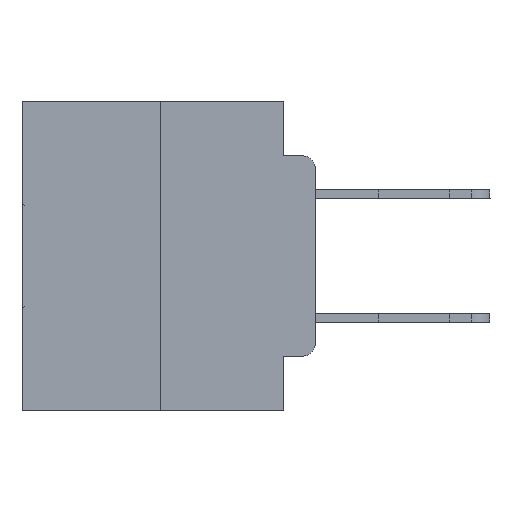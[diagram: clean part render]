
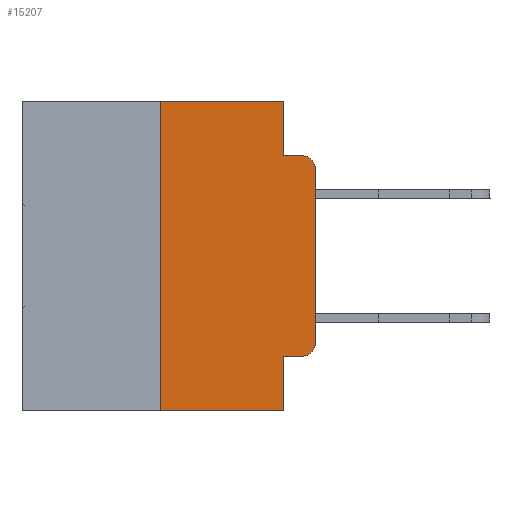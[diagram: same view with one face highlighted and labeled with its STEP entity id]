
A CAD part, left-side view. The second image highlights one B-rep face of the part: STEP entity #15207.
In plain terms, the highlighted planar face has unit normal (-1, 0, 0).
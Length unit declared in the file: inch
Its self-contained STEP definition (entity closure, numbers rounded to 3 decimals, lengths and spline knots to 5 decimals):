
#726 = DIRECTION ( 'NONE',  ( 0., 0., -1. ) ) ;
#745 = ORIENTED_EDGE ( 'NONE', *, *, #25341, .F. ) ;
#1807 = CARTESIAN_POINT ( 'NONE',  ( 0., 0.25, 0. ) ) ;
#2274 = ORIENTED_EDGE ( 'NONE', *, *, #5739, .F. ) ;
#2946 = VECTOR ( 'NONE', #726, 39.37008 ) ;
#3350 = CARTESIAN_POINT ( 'NONE',  ( 0., 0., 0. ) ) ;
#3655 = VECTOR ( 'NONE', #16462, 39.37008 ) ;
#3758 = VERTEX_POINT ( 'NONE', #6797 ) ;
#4057 = EDGE_CURVE ( 'NONE', #8524, #8776, #22356, .T. ) ;
#4253 = LINE ( 'NONE', #29282, #29813 ) ;
#4266 = VERTEX_POINT ( 'NONE', #20864 ) ;
#4558 = EDGE_LOOP ( 'NONE', ( #22821, #4998, #11525, #25002, #745, #2274, #21728, #22476, #28677, #23927 ) ) ;
#4998 = ORIENTED_EDGE ( 'NONE', *, *, #12325, .T. ) ;
#5038 = VECTOR ( 'NONE', #22798, 39.37008 ) ;
#5739 = EDGE_CURVE ( 'NONE', #27080, #23513, #28516, .T. ) ;
#6314 = VERTEX_POINT ( 'NONE', #9433 ) ;
#6797 = CARTESIAN_POINT ( 'NONE',  ( 0., 0., -0.1085 ) ) ;
#6836 = AXIS2_PLACEMENT_3D ( 'NONE', #23693, #9259, #26012 ) ;
#7069 = LINE ( 'NONE', #26354, #19217 ) ;
#7763 = DIRECTION ( 'NONE',  ( 0., 0., -1. ) ) ;
#7784 = CIRCLE ( 'NONE', #6836, 0.02 ) ;
#8524 = VERTEX_POINT ( 'NONE', #25111 ) ;
#8709 = CARTESIAN_POINT ( 'NONE',  ( 0., 0.051, -0.0885 ) ) ;
#8776 = VERTEX_POINT ( 'NONE', #26008 ) ;
#9035 = EDGE_CURVE ( 'NONE', #16711, #6314, #4253, .T. ) ;
#9223 = AXIS2_PLACEMENT_3D ( 'NONE', #10762, #13210, #29814 ) ;
#9259 = DIRECTION ( 'NONE',  ( -1., 0., 0. ) ) ;
#9404 = DIRECTION ( 'NONE',  ( 0., -1., 0. ) ) ;
#9433 = CARTESIAN_POINT ( 'NONE',  ( 0., 0.051, -0.0885 ) ) ;
#10379 = VERTEX_POINT ( 'NONE', #17239 ) ;
#10684 = EDGE_CURVE ( 'NONE', #6314, #4266, #16758, .T. ) ;
#10762 = CARTESIAN_POINT ( 'NONE',  ( 0., 0.473, 0. ) ) ;
#11124 = CARTESIAN_POINT ( 'NONE',  ( 0., 0.051, 0. ) ) ;
#11525 = ORIENTED_EDGE ( 'NONE', *, *, #10684, .F. ) ;
#12325 = EDGE_CURVE ( 'NONE', #3758, #4266, #22347, .T. ) ;
#12922 = DIRECTION ( 'NONE',  ( -1., 0., 0. ) ) ;
#13210 = DIRECTION ( 'NONE',  ( 1., 0., 0. ) ) ;
#14292 = CARTESIAN_POINT ( 'NONE',  ( 0., 0.473, -0.5 ) ) ;
#15207 = ADVANCED_FACE ( 'NONE', ( #30270 ), #15519, .F. ) ;
#15519 = PLANE ( 'NONE',  #9223 ) ;
#15844 = CARTESIAN_POINT ( 'NONE',  ( 0., 0.25, 0. ) ) ;
#16055 = CARTESIAN_POINT ( 'NONE',  ( 0., 0.051, -0.4115 ) ) ;
#16462 = DIRECTION ( 'NONE',  ( 0., 0., 1. ) ) ;
#16711 = VERTEX_POINT ( 'NONE', #11124 ) ;
#16758 = LINE ( 'NONE', #8709, #27145 ) ;
#17174 = EDGE_CURVE ( 'NONE', #10379, #3758, #30533, .T. ) ;
#17239 = CARTESIAN_POINT ( 'NONE',  ( 0., 0., -0.3915 ) ) ;
#17476 = VECTOR ( 'NONE', #9404, 39.37008 ) ;
#19211 = EDGE_CURVE ( 'NONE', #27080, #8776, #30023, .T. ) ;
#19217 = VECTOR ( 'NONE', #28713, 39.37008 ) ;
#20811 = AXIS2_PLACEMENT_3D ( 'NONE', #26765, #12922, #29520 ) ;
#20864 = CARTESIAN_POINT ( 'NONE',  ( 0., 0.02, -0.0885 ) ) ;
#21728 = ORIENTED_EDGE ( 'NONE', *, *, #19211, .T. ) ;
#22347 = CIRCLE ( 'NONE', #20811, 0.02 ) ;
#22356 = LINE ( 'NONE', #24877, #2946 ) ;
#22476 = ORIENTED_EDGE ( 'NONE', *, *, #4057, .F. ) ;
#22798 = DIRECTION ( 'NONE',  ( 0., 0., 1. ) ) ;
#22821 = ORIENTED_EDGE ( 'NONE', *, *, #17174, .T. ) ;
#23177 = DIRECTION ( 'NONE',  ( 0., -1., 0. ) ) ;
#23280 = DIRECTION ( 'NONE',  ( 0., -1., 0. ) ) ;
#23513 = VERTEX_POINT ( 'NONE', #15844 ) ;
#23693 = CARTESIAN_POINT ( 'NONE',  ( 0., 0.02, -0.3915 ) ) ;
#23789 = CARTESIAN_POINT ( 'NONE',  ( 0., 0.02, -0.4115 ) ) ;
#23927 = ORIENTED_EDGE ( 'NONE', *, *, #28851, .T. ) ;
#24247 = VECTOR ( 'NONE', #23280, 39.37008 ) ;
#24877 = CARTESIAN_POINT ( 'NONE',  ( 0., 0.051, 0. ) ) ;
#25002 = ORIENTED_EDGE ( 'NONE', *, *, #9035, .F. ) ;
#25111 = CARTESIAN_POINT ( 'NONE',  ( 0., 0.051, -0.4115 ) ) ;
#25341 = EDGE_CURVE ( 'NONE', #23513, #16711, #7069, .T. ) ;
#25878 = CARTESIAN_POINT ( 'NONE',  ( 0., 0.25, -0.5 ) ) ;
#26008 = CARTESIAN_POINT ( 'NONE',  ( 0., 0.051, -0.5 ) ) ;
#26012 = DIRECTION ( 'NONE',  ( 0., 0., -1. ) ) ;
#26354 = CARTESIAN_POINT ( 'NONE',  ( 0., 0.473, 0. ) ) ;
#26765 = CARTESIAN_POINT ( 'NONE',  ( 0., 0.02, -0.1085 ) ) ;
#27080 = VERTEX_POINT ( 'NONE', #25878 ) ;
#27145 = VECTOR ( 'NONE', #23177, 39.37008 ) ;
#28516 = LINE ( 'NONE', #1807, #3655 ) ;
#28677 = ORIENTED_EDGE ( 'NONE', *, *, #30417, .T. ) ;
#28713 = DIRECTION ( 'NONE',  ( 0., -1., 0. ) ) ;
#28851 = EDGE_CURVE ( 'NONE', #28881, #10379, #7784, .T. ) ;
#28881 = VERTEX_POINT ( 'NONE', #23789 ) ;
#29282 = CARTESIAN_POINT ( 'NONE',  ( 0., 0.051, 0. ) ) ;
#29520 = DIRECTION ( 'NONE',  ( 0., 0., -1. ) ) ;
#29813 = VECTOR ( 'NONE', #7763, 39.37008 ) ;
#29814 = DIRECTION ( 'NONE',  ( 0., 0., -1. ) ) ;
#30023 = LINE ( 'NONE', #14292, #17476 ) ;
#30270 = FACE_OUTER_BOUND ( 'NONE', #4558, .T. ) ;
#30417 = EDGE_CURVE ( 'NONE', #8524, #28881, #30456, .T. ) ;
#30456 = LINE ( 'NONE', #16055, #24247 ) ;
#30533 = LINE ( 'NONE', #3350, #5038 ) ;
